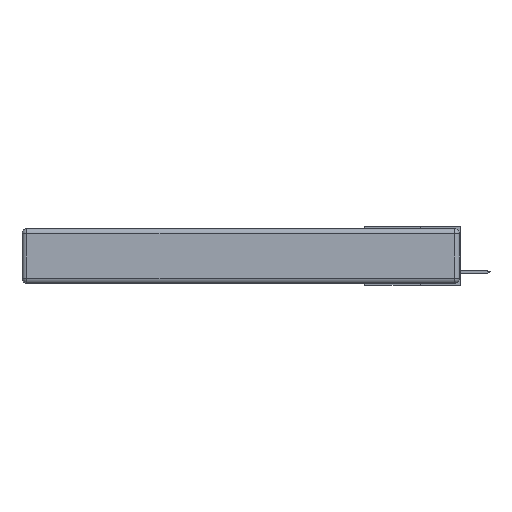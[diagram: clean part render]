
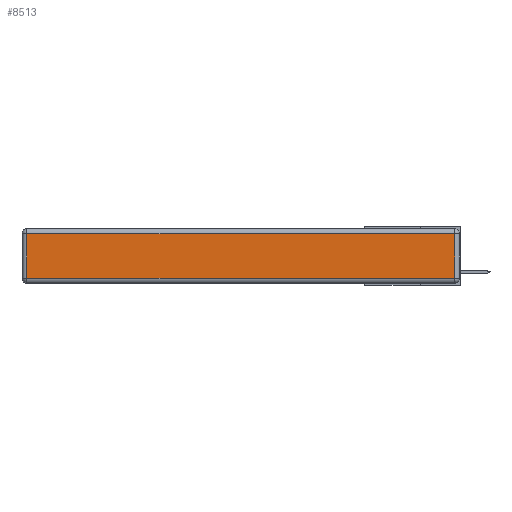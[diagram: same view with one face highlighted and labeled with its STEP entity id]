
A CAD part, left-side view. The second image highlights one B-rep face of the part: STEP entity #8513.
In plain terms, the highlighted planar face has unit normal (-1, 0, 0).
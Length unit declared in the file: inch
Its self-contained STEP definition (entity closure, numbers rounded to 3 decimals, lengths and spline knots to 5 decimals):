
#121 = LINE ( 'NONE', #3378, #7634 ) ;
#668 = CARTESIAN_POINT ( 'NONE',  ( 0., 0., -0.343 ) ) ;
#1252 = VERTEX_POINT ( 'NONE', #2600 ) ;
#1561 = DIRECTION ( 'NONE',  ( 0., 0., -1. ) ) ;
#1633 = CARTESIAN_POINT ( 'NONE',  ( 0., 2.72, -0.313 ) ) ;
#2122 = LINE ( 'NONE', #3660, #5529 ) ;
#2207 = EDGE_LOOP ( 'NONE', ( #3997, #2272, #10671, #11735 ) ) ;
#2272 = ORIENTED_EDGE ( 'NONE', *, *, #4700, .T. ) ;
#2507 = EDGE_CURVE ( 'NONE', #4130, #1252, #121, .T. ) ;
#2579 = DIRECTION ( 'NONE',  ( 0., 0., 1. ) ) ;
#2587 = DIRECTION ( 'NONE',  ( 0., 0., 1. ) ) ;
#2600 = CARTESIAN_POINT ( 'NONE',  ( 0., 0.03, -0.313 ) ) ;
#2607 = EDGE_CURVE ( 'NONE', #9109, #4461, #11282, .T. ) ;
#2952 = DIRECTION ( 'NONE',  ( 0., 1., 0. ) ) ;
#3378 = CARTESIAN_POINT ( 'NONE',  ( 0., 0., -0.313 ) ) ;
#3660 = CARTESIAN_POINT ( 'NONE',  ( 0., 0.03, -0.343 ) ) ;
#3997 = ORIENTED_EDGE ( 'NONE', *, *, #2507, .T. ) ;
#4130 = VERTEX_POINT ( 'NONE', #1633 ) ;
#4461 = VERTEX_POINT ( 'NONE', #7962 ) ;
#4700 = EDGE_CURVE ( 'NONE', #1252, #9109, #2122, .T. ) ;
#5225 = AXIS2_PLACEMENT_3D ( 'NONE', #668, #9476, #2587 ) ;
#5529 = VECTOR ( 'NONE', #2579, 39.37008 ) ;
#6559 = PLANE ( 'NONE',  #5225 ) ;
#7475 = VECTOR ( 'NONE', #2952, 39.37008 ) ;
#7634 = VECTOR ( 'NONE', #10266, 39.37008 ) ;
#7943 = EDGE_CURVE ( 'NONE', #4461, #4130, #8793, .T. ) ;
#7962 = CARTESIAN_POINT ( 'NONE',  ( 0., 2.72, -0.03 ) ) ;
#7997 = CARTESIAN_POINT ( 'NONE',  ( 0., 0.03, -0.03 ) ) ;
#8354 = CARTESIAN_POINT ( 'NONE',  ( 0., 2.72, -0.343 ) ) ;
#8513 = ADVANCED_FACE ( 'NONE', ( #9228 ), #6559, .T. ) ;
#8793 = LINE ( 'NONE', #8354, #9096 ) ;
#9096 = VECTOR ( 'NONE', #1561, 39.37008 ) ;
#9109 = VERTEX_POINT ( 'NONE', #7997 ) ;
#9228 = FACE_OUTER_BOUND ( 'NONE', #2207, .T. ) ;
#9476 = DIRECTION ( 'NONE',  ( -1., 0., 0. ) ) ;
#9918 = CARTESIAN_POINT ( 'NONE',  ( 0., 2.75, -0.03 ) ) ;
#10266 = DIRECTION ( 'NONE',  ( 0., -1., 0. ) ) ;
#10671 = ORIENTED_EDGE ( 'NONE', *, *, #2607, .T. ) ;
#11282 = LINE ( 'NONE', #9918, #7475 ) ;
#11735 = ORIENTED_EDGE ( 'NONE', *, *, #7943, .T. ) ;
